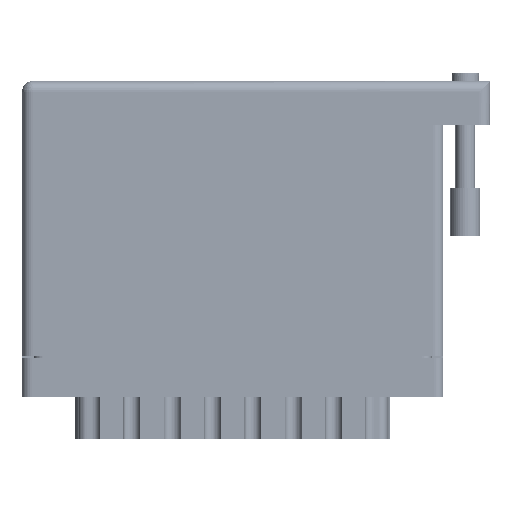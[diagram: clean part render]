
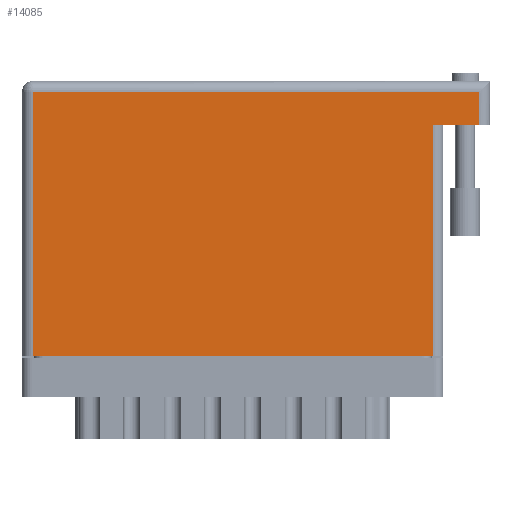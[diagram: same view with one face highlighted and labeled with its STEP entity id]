
A CAD part, front view. The second image highlights one B-rep face of the part: STEP entity #14085.
In plain terms, the highlighted face is planar.
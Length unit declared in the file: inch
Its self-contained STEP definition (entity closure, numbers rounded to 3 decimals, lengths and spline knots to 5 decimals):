
#1004 = ORIENTED_EDGE ( 'NONE', *, *, #40054, .T. ) ;
#3275 = CARTESIAN_POINT ( 'NONE',  ( 2.948, 1.495, 0. ) ) ;
#3412 = LINE ( 'NONE', #12303, #23540 ) ;
#3568 = ORIENTED_EDGE ( 'NONE', *, *, #6132, .T. ) ;
#4966 = CARTESIAN_POINT ( 'NONE',  ( 3.018, 1.495, 0. ) ) ;
#6132 = EDGE_CURVE ( 'NONE', #53861, #25233, #45903, .T. ) ;
#6312 = AXIS2_PLACEMENT_3D ( 'NONE', #20442, #8690, #71254 ) ;
#6862 = LINE ( 'NONE', #4966, #42053 ) ;
#8690 = DIRECTION ( 'NONE',  ( 0., 0., -1. ) ) ;
#9557 = EDGE_CURVE ( 'NONE', #63638, #67598, #16091, .T. ) ;
#10997 = LINE ( 'NONE', #21469, #65483 ) ;
#11472 = DIRECTION ( 'NONE',  ( 1., 0., 0. ) ) ;
#12303 = CARTESIAN_POINT ( 'NONE',  ( 2.948, 1.775, 0. ) ) ;
#14085 = ADVANCED_FACE ( 'NONE', ( #19881 ), #48430, .F. ) ;
#14093 = LINE ( 'NONE', #45138, #55400 ) ;
#15474 = VERTEX_POINT ( 'NONE', #55229 ) ;
#15725 = CARTESIAN_POINT ( 'NONE',  ( 2.648, 1.495, 0. ) ) ;
#16091 = LINE ( 'NONE', #24887, #61732 ) ;
#19881 = FACE_OUTER_BOUND ( 'NONE', #70458, .T. ) ;
#20442 = CARTESIAN_POINT ( 'NONE',  ( 0., 1.775, 0. ) ) ;
#21469 = CARTESIAN_POINT ( 'NONE',  ( 0., 1.705, 0. ) ) ;
#21689 = ORIENTED_EDGE ( 'NONE', *, *, #9557, .T. ) ;
#23250 = DIRECTION ( 'NONE',  ( 0., -1., 0. ) ) ;
#23540 = VECTOR ( 'NONE', #52566, 39.37008 ) ;
#24188 = VERTEX_POINT ( 'NONE', #3275 ) ;
#24887 = CARTESIAN_POINT ( 'NONE',  ( 2.648, 1.495, 0. ) ) ;
#25233 = VERTEX_POINT ( 'NONE', #69609 ) ;
#25564 = ORIENTED_EDGE ( 'NONE', *, *, #37018, .T. ) ;
#26896 = ORIENTED_EDGE ( 'NONE', *, *, #33334, .T. ) ;
#28175 = CARTESIAN_POINT ( 'NONE',  ( 0.07, 0., 0. ) ) ;
#31795 = CARTESIAN_POINT ( 'NONE',  ( 2.648, 0., 0. ) ) ;
#31884 = VECTOR ( 'NONE', #23250, 39.37008 ) ;
#33334 = EDGE_CURVE ( 'NONE', #24188, #15474, #3412, .T. ) ;
#37018 = EDGE_CURVE ( 'NONE', #25233, #63638, #14093, .T. ) ;
#40054 = EDGE_CURVE ( 'NONE', #15474, #53861, #10997, .T. ) ;
#42053 = VECTOR ( 'NONE', #49826, 39.37008 ) ;
#45138 = CARTESIAN_POINT ( 'NONE',  ( 0., 0., 0. ) ) ;
#45903 = LINE ( 'NONE', #28175, #31884 ) ;
#47318 = EDGE_CURVE ( 'NONE', #24188, #67598, #6862, .T. ) ;
#48430 = PLANE ( 'NONE',  #6312 ) ;
#49826 = DIRECTION ( 'NONE',  ( -1., 0., 0. ) ) ;
#52566 = DIRECTION ( 'NONE',  ( 0., 1., 0. ) ) ;
#53861 = VERTEX_POINT ( 'NONE', #56088 ) ;
#54346 = ORIENTED_EDGE ( 'NONE', *, *, #47318, .F. ) ;
#55229 = CARTESIAN_POINT ( 'NONE',  ( 2.948, 1.705, 0. ) ) ;
#55400 = VECTOR ( 'NONE', #11472, 39.37008 ) ;
#56088 = CARTESIAN_POINT ( 'NONE',  ( 0.07, 1.705, 0. ) ) ;
#59040 = DIRECTION ( 'NONE',  ( 0., 1., 0. ) ) ;
#59802 = DIRECTION ( 'NONE',  ( -1., 0., 0. ) ) ;
#61732 = VECTOR ( 'NONE', #59040, 39.37008 ) ;
#63638 = VERTEX_POINT ( 'NONE', #31795 ) ;
#65483 = VECTOR ( 'NONE', #59802, 39.37008 ) ;
#67598 = VERTEX_POINT ( 'NONE', #15725 ) ;
#69609 = CARTESIAN_POINT ( 'NONE',  ( 0.07, 0., 0. ) ) ;
#70458 = EDGE_LOOP ( 'NONE', ( #25564, #21689, #54346, #26896, #1004, #3568 ) ) ;
#71254 = DIRECTION ( 'NONE',  ( -1., 0., 0. ) ) ;
